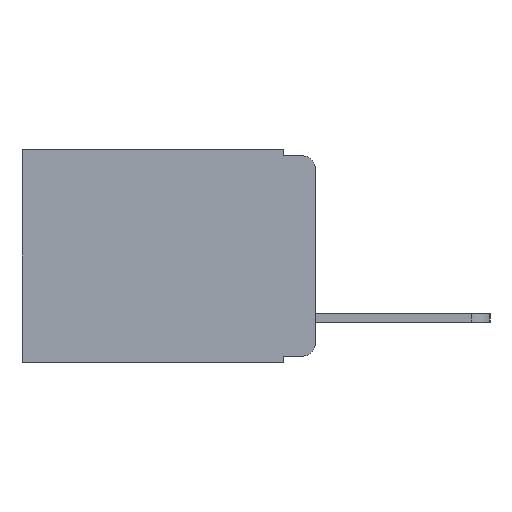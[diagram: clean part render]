
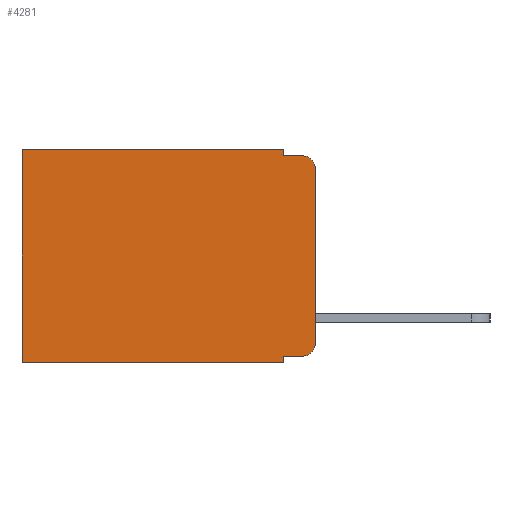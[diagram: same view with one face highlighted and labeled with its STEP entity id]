
A CAD part, left-side view. The second image highlights one B-rep face of the part: STEP entity #4281.
In plain terms, the highlighted planar face has unit normal (-1, 0, 0).
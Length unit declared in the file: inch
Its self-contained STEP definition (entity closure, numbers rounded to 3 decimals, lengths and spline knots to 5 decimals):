
#292 = CARTESIAN_POINT ( 'NONE',  ( 0.298, 0.02, -0.313 ) ) ;
#339 = AXIS2_PLACEMENT_3D ( 'NONE', #2116, #4800, #13261 ) ;
#348 = DIRECTION ( 'NONE',  ( -1., 0., 0. ) ) ;
#399 = DIRECTION ( 'NONE',  ( 0., 0., -1. ) ) ;
#409 = ORIENTED_EDGE ( 'NONE', *, *, #6735, .F. ) ;
#582 = VERTEX_POINT ( 'NONE', #815 ) ;
#639 = ORIENTED_EDGE ( 'NONE', *, *, #8859, .T. ) ;
#815 = CARTESIAN_POINT ( 'NONE',  ( 0.298, 0.051, 0. ) ) ;
#938 = CARTESIAN_POINT ( 'NONE',  ( 0.298, 0.473, 0. ) ) ;
#1262 = VERTEX_POINT ( 'NONE', #6384 ) ;
#2116 = CARTESIAN_POINT ( 'NONE',  ( 0.298, 0., 0. ) ) ;
#2202 = VECTOR ( 'NONE', #7775, 39.37008 ) ;
#2215 = CARTESIAN_POINT ( 'NONE',  ( 0.298, 0.02, -0.01 ) ) ;
#2258 = VERTEX_POINT ( 'NONE', #12113 ) ;
#2429 = DIRECTION ( 'NONE',  ( 0., -1., 0. ) ) ;
#2458 = DIRECTION ( 'NONE',  ( 0., 0., -1. ) ) ;
#2470 = CARTESIAN_POINT ( 'NONE',  ( 0.298, 0.051, 0. ) ) ;
#2998 = VERTEX_POINT ( 'NONE', #7980 ) ;
#3284 = LINE ( 'NONE', #16062, #12873 ) ;
#3584 = DIRECTION ( 'NONE',  ( 0., 1., 0. ) ) ;
#3712 = VERTEX_POINT ( 'NONE', #15382 ) ;
#3792 = LINE ( 'NONE', #5070, #16093 ) ;
#3834 = CARTESIAN_POINT ( 'NONE',  ( 0.298, 0.473, 0. ) ) ;
#3845 = CARTESIAN_POINT ( 'NONE',  ( 0.298, 0.02, -0.03 ) ) ;
#4010 = LINE ( 'NONE', #12657, #15534 ) ;
#4281 = ADVANCED_FACE ( 'NONE', ( #11743 ), #16297, .F. ) ;
#4468 = VERTEX_POINT ( 'NONE', #7763 ) ;
#4729 = AXIS2_PLACEMENT_3D ( 'NONE', #292, #348, #399 ) ;
#4755 = EDGE_CURVE ( 'NONE', #4468, #5879, #12779, .T. ) ;
#4800 = DIRECTION ( 'NONE',  ( 1., 0., 0. ) ) ;
#5070 = CARTESIAN_POINT ( 'NONE',  ( 0.298, 0., 0. ) ) ;
#5519 = DIRECTION ( 'NONE',  ( 0., 0., -1. ) ) ;
#5572 = ORIENTED_EDGE ( 'NONE', *, *, #13065, .T. ) ;
#5585 = ORIENTED_EDGE ( 'NONE', *, *, #10799, .F. ) ;
#5651 = EDGE_CURVE ( 'NONE', #4468, #1262, #3792, .T. ) ;
#5759 = LINE ( 'NONE', #14016, #12341 ) ;
#5879 = VERTEX_POINT ( 'NONE', #2215 ) ;
#6222 = CARTESIAN_POINT ( 'NONE',  ( 0.298, 0.473, -0.343 ) ) ;
#6280 = VERTEX_POINT ( 'NONE', #6222 ) ;
#6384 = CARTESIAN_POINT ( 'NONE',  ( 0.298, 0., -0.313 ) ) ;
#6407 = EDGE_CURVE ( 'NONE', #7973, #1262, #8978, .T. ) ;
#6735 = EDGE_CURVE ( 'NONE', #2998, #6280, #4010, .T. ) ;
#6843 = DIRECTION ( 'NONE',  ( 0., 1., 0. ) ) ;
#7109 = LINE ( 'NONE', #938, #2202 ) ;
#7467 = ORIENTED_EDGE ( 'NONE', *, *, #6407, .T. ) ;
#7763 = CARTESIAN_POINT ( 'NONE',  ( 0.298, 0., -0.03 ) ) ;
#7775 = DIRECTION ( 'NONE',  ( 0., 0., -1. ) ) ;
#7973 = VERTEX_POINT ( 'NONE', #8953 ) ;
#7980 = CARTESIAN_POINT ( 'NONE',  ( 0.298, 0.051, -0.343 ) ) ;
#8069 = VECTOR ( 'NONE', #14179, 39.37008 ) ;
#8630 = ORIENTED_EDGE ( 'NONE', *, *, #4755, .T. ) ;
#8650 = VECTOR ( 'NONE', #15043, 39.37008 ) ;
#8822 = AXIS2_PLACEMENT_3D ( 'NONE', #3845, #11454, #2458 ) ;
#8859 = EDGE_CURVE ( 'NONE', #582, #13112, #14324, .T. ) ;
#8953 = CARTESIAN_POINT ( 'NONE',  ( 0.298, 0.02, -0.333 ) ) ;
#8978 = CIRCLE ( 'NONE', #4729, 0.02 ) ;
#9995 = EDGE_CURVE ( 'NONE', #3712, #2998, #5759, .T. ) ;
#10787 = DIRECTION ( 'NONE',  ( 0., 0., -1. ) ) ;
#10799 = EDGE_CURVE ( 'NONE', #582, #2258, #11779, .T. ) ;
#10843 = CARTESIAN_POINT ( 'NONE',  ( 0.298, 0.051, -0.333 ) ) ;
#11260 = LINE ( 'NONE', #10843, #8069 ) ;
#11313 = VECTOR ( 'NONE', #6843, 39.37008 ) ;
#11454 = DIRECTION ( 'NONE',  ( -1., 0., 0. ) ) ;
#11743 = FACE_OUTER_BOUND ( 'NONE', #14660, .T. ) ;
#11779 = LINE ( 'NONE', #2470, #8650 ) ;
#12113 = CARTESIAN_POINT ( 'NONE',  ( 0.298, 0.051, -0.01 ) ) ;
#12116 = ORIENTED_EDGE ( 'NONE', *, *, #14598, .T. ) ;
#12318 = ORIENTED_EDGE ( 'NONE', *, *, #5651, .F. ) ;
#12341 = VECTOR ( 'NONE', #5519, 39.37008 ) ;
#12657 = CARTESIAN_POINT ( 'NONE',  ( 0.298, 0., -0.343 ) ) ;
#12779 = CIRCLE ( 'NONE', #8822, 0.02 ) ;
#12873 = VECTOR ( 'NONE', #2429, 39.37008 ) ;
#12882 = ORIENTED_EDGE ( 'NONE', *, *, #9995, .F. ) ;
#13065 = EDGE_CURVE ( 'NONE', #13112, #6280, #7109, .T. ) ;
#13112 = VERTEX_POINT ( 'NONE', #3834 ) ;
#13261 = DIRECTION ( 'NONE',  ( 0., 0., -1. ) ) ;
#13307 = ORIENTED_EDGE ( 'NONE', *, *, #13790, .F. ) ;
#13790 = EDGE_CURVE ( 'NONE', #2258, #5879, #3284, .T. ) ;
#14016 = CARTESIAN_POINT ( 'NONE',  ( 0.298, 0.051, 0. ) ) ;
#14179 = DIRECTION ( 'NONE',  ( 0., -1., 0. ) ) ;
#14324 = LINE ( 'NONE', #15341, #11313 ) ;
#14598 = EDGE_CURVE ( 'NONE', #3712, #7973, #11260, .T. ) ;
#14660 = EDGE_LOOP ( 'NONE', ( #12318, #8630, #13307, #5585, #639, #5572, #409, #12882, #12116, #7467 ) ) ;
#15043 = DIRECTION ( 'NONE',  ( 0., 0., -1. ) ) ;
#15341 = CARTESIAN_POINT ( 'NONE',  ( 0.298, 0., 0. ) ) ;
#15382 = CARTESIAN_POINT ( 'NONE',  ( 0.298, 0.051, -0.333 ) ) ;
#15534 = VECTOR ( 'NONE', #3584, 39.37008 ) ;
#16062 = CARTESIAN_POINT ( 'NONE',  ( 0.298, 0.051, -0.01 ) ) ;
#16093 = VECTOR ( 'NONE', #10787, 39.37008 ) ;
#16297 = PLANE ( 'NONE',  #339 ) ;
